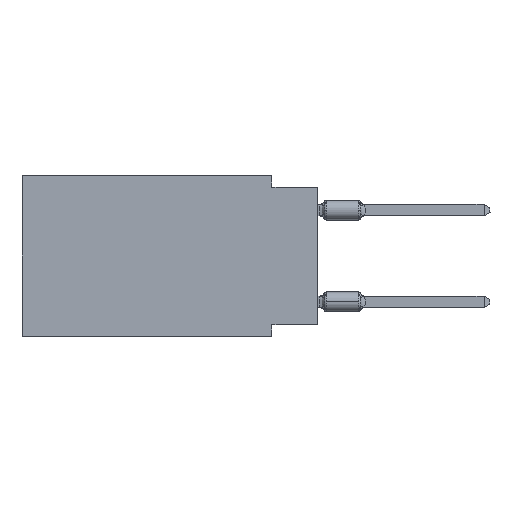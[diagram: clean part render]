
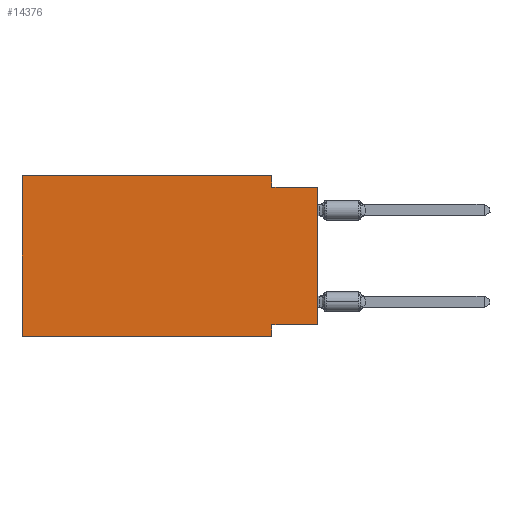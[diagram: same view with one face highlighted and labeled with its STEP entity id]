
A CAD part, left-side view. The second image highlights one B-rep face of the part: STEP entity #14376.
In plain terms, the highlighted planar face has unit normal (-1, 0, 0).
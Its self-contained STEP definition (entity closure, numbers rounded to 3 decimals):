
#1811 = VECTOR ( 'NONE', #22260, 1000. ) ;
#2346 = VERTEX_POINT ( 'NONE', #29822 ) ;
#4158 = CARTESIAN_POINT ( 'NONE',  ( 0., 16.383, -8.89 ) ) ;
#4809 = CARTESIAN_POINT ( 'NONE',  ( 0., 0., -0.635 ) ) ;
#5445 = CARTESIAN_POINT ( 'NONE',  ( 0., 16.383, -8.89 ) ) ;
#5702 = FACE_OUTER_BOUND ( 'NONE', #45373, .T. ) ;
#5876 = CARTESIAN_POINT ( 'NONE',  ( 0., 2.54, 0. ) ) ;
#6511 = LINE ( 'NONE', #23416, #51691 ) ;
#6604 = CARTESIAN_POINT ( 'NONE',  ( 0., 2.54, 0. ) ) ;
#6678 = ORIENTED_EDGE ( 'NONE', *, *, #11462, .T. ) ;
#7609 = DIRECTION ( 'NONE',  ( 0., -1., 0. ) ) ;
#7938 = VECTOR ( 'NONE', #7609, 1000. ) ;
#10040 = EDGE_CURVE ( 'NONE', #10233, #16144, #40965, .T. ) ;
#10233 = VERTEX_POINT ( 'NONE', #36128 ) ;
#10774 = VERTEX_POINT ( 'NONE', #50974 ) ;
#11462 = EDGE_CURVE ( 'NONE', #2346, #16144, #33412, .T. ) ;
#13419 = ORIENTED_EDGE ( 'NONE', *, *, #10040, .F. ) ;
#13589 = CARTESIAN_POINT ( 'NONE',  ( 0., 0., 0. ) ) ;
#13771 = VERTEX_POINT ( 'NONE', #6604 ) ;
#14376 = ADVANCED_FACE ( 'NONE', ( #5702 ), #49242, .F. ) ;
#14666 = VECTOR ( 'NONE', #24228, 1000. ) ;
#15626 = VECTOR ( 'NONE', #19457, 1000. ) ;
#16144 = VERTEX_POINT ( 'NONE', #19207 ) ;
#16876 = EDGE_CURVE ( 'NONE', #10774, #19364, #33096, .T. ) ;
#17419 = VERTEX_POINT ( 'NONE', #50652 ) ;
#17849 = DIRECTION ( 'NONE',  ( 0., 0., -1. ) ) ;
#19207 = CARTESIAN_POINT ( 'NONE',  ( 0., 0., -0.635 ) ) ;
#19364 = VERTEX_POINT ( 'NONE', #29048 ) ;
#19401 = ORIENTED_EDGE ( 'NONE', *, *, #16876, .F. ) ;
#19457 = DIRECTION ( 'NONE',  ( 0., -1., 0. ) ) ;
#22260 = DIRECTION ( 'NONE',  ( 0., 0., -1. ) ) ;
#22365 = EDGE_CURVE ( 'NONE', #17419, #13771, #51106, .T. ) ;
#23246 = ORIENTED_EDGE ( 'NONE', *, *, #42795, .F. ) ;
#23416 = CARTESIAN_POINT ( 'NONE',  ( 0., 16.383, 0. ) ) ;
#23546 = VECTOR ( 'NONE', #42703, 1000. ) ;
#24228 = DIRECTION ( 'NONE',  ( 0., -1., 0. ) ) ;
#25354 = EDGE_CURVE ( 'NONE', #36131, #17419, #6511, .T. ) ;
#25767 = DIRECTION ( 'NONE',  ( 1., 0., 0. ) ) ;
#26116 = CARTESIAN_POINT ( 'NONE',  ( 0., 0., -8.255 ) ) ;
#27150 = EDGE_CURVE ( 'NONE', #2346, #10774, #46655, .T. ) ;
#27639 = VECTOR ( 'NONE', #50718, 1000. ) ;
#29048 = CARTESIAN_POINT ( 'NONE',  ( 0., 2.54, -8.89 ) ) ;
#29822 = CARTESIAN_POINT ( 'NONE',  ( 0., 0., -8.255 ) ) ;
#30181 = CARTESIAN_POINT ( 'NONE',  ( 0., 2.54, -8.89 ) ) ;
#31593 = CARTESIAN_POINT ( 'NONE',  ( 0., 16.383, 0. ) ) ;
#32189 = ORIENTED_EDGE ( 'NONE', *, *, #22365, .F. ) ;
#32473 = ORIENTED_EDGE ( 'NONE', *, *, #25354, .F. ) ;
#33096 = LINE ( 'NONE', #30181, #1811 ) ;
#33412 = LINE ( 'NONE', #13589, #38124 ) ;
#34637 = LINE ( 'NONE', #5876, #27639 ) ;
#35907 = AXIS2_PLACEMENT_3D ( 'NONE', #37648, #25767, #17849 ) ;
#36128 = CARTESIAN_POINT ( 'NONE',  ( 0., 2.54, -0.635 ) ) ;
#36131 = VERTEX_POINT ( 'NONE', #5445 ) ;
#37648 = CARTESIAN_POINT ( 'NONE',  ( 0., 16.383, 0. ) ) ;
#38124 = VECTOR ( 'NONE', #45771, 1000. ) ;
#40933 = ORIENTED_EDGE ( 'NONE', *, *, #50396, .T. ) ;
#40965 = LINE ( 'NONE', #4809, #7938 ) ;
#42703 = DIRECTION ( 'NONE',  ( 0., 1., 0. ) ) ;
#42795 = EDGE_CURVE ( 'NONE', #13771, #10233, #34637, .T. ) ;
#43742 = ORIENTED_EDGE ( 'NONE', *, *, #27150, .F. ) ;
#45373 = EDGE_LOOP ( 'NONE', ( #6678, #13419, #23246, #32189, #32473, #40933, #19401, #43742 ) ) ;
#45771 = DIRECTION ( 'NONE',  ( 0., 0., 1. ) ) ;
#46655 = LINE ( 'NONE', #26116, #23546 ) ;
#47861 = LINE ( 'NONE', #4158, #14666 ) ;
#49242 = PLANE ( 'NONE',  #35907 ) ;
#50396 = EDGE_CURVE ( 'NONE', #36131, #19364, #47861, .T. ) ;
#50652 = CARTESIAN_POINT ( 'NONE',  ( 0., 16.383, 0. ) ) ;
#50718 = DIRECTION ( 'NONE',  ( 0., 0., -1. ) ) ;
#50974 = CARTESIAN_POINT ( 'NONE',  ( 0., 2.54, -8.255 ) ) ;
#51106 = LINE ( 'NONE', #31593, #15626 ) ;
#51618 = DIRECTION ( 'NONE',  ( 0., 0., 1. ) ) ;
#51691 = VECTOR ( 'NONE', #51618, 1000. ) ;
